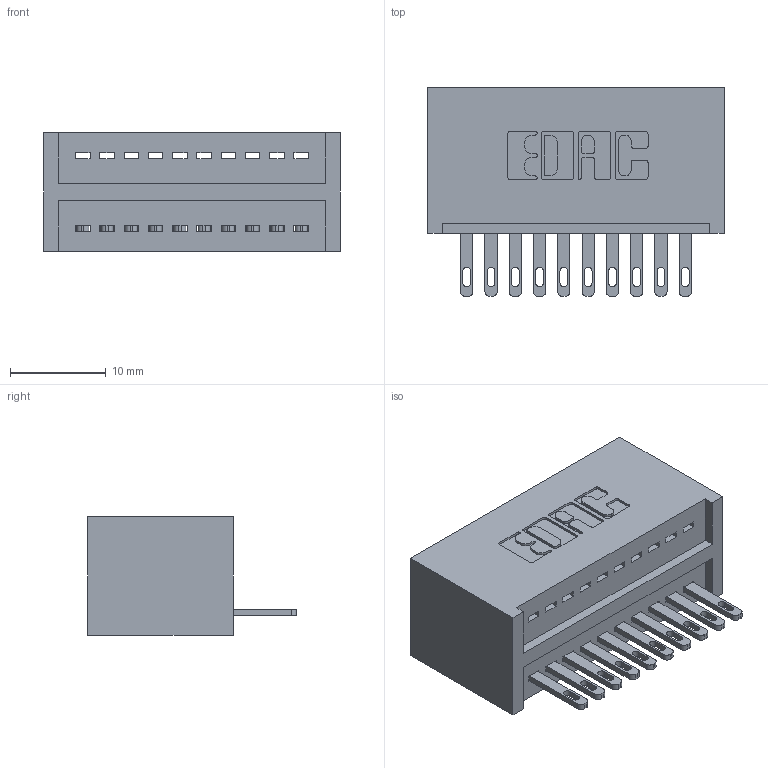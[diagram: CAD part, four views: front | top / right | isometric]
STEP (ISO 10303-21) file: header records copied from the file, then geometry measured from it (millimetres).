
FILE_DESCRIPTION (( 'STEP AP203' ), '1' );
FILE_NAME ('325-010-500-101.STEP', '2020-02-24T15:01:08', ( '' ), ( '' ), 'SwSTEP 2.0', 'SolidWorks 2016', '' );
FILE_SCHEMA (( 'CONFIG_CONTROL_DESIGN' ));
Length unit declared in the file: inch
Products named in the file (3): 325-292-001_325-293-100; 325 Part_Lugless; 325-010-500-101
Assembly tree (11 placements, depth 2):
  325-010-500-101
    325 Part_Lugless
    325-292-001_325-293-100  x10
Bounding box: 31.04 x 21.84 x 12.45 mm (x, y, z)
Volume: 4266.6 mm3; surface area: 4632.2 mm2
Topology: 11 solids, 11 shells, 646 faces, 1967 edges, 1310 vertices
Faces by surface type: plane 426, cylinder 220
Entity records: 9905 total; most frequent: CARTESIAN_POINT 1720, ORIENTED_EDGE 1666, DIRECTION 1509, EDGE_CURVE 833, LINE 709, VECTOR 709, VERTEX_POINT 554, AXIS2_PLACEMENT_3D 400
